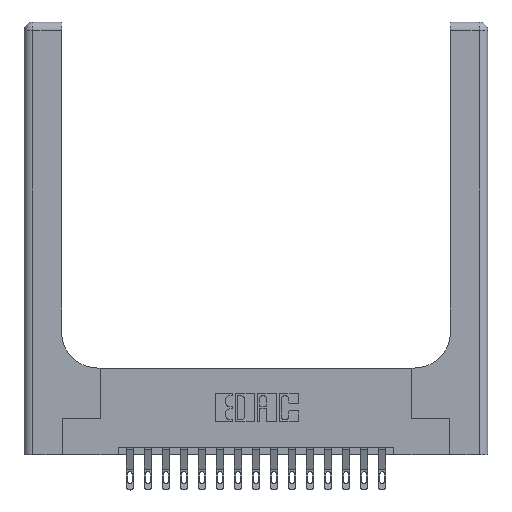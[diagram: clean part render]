
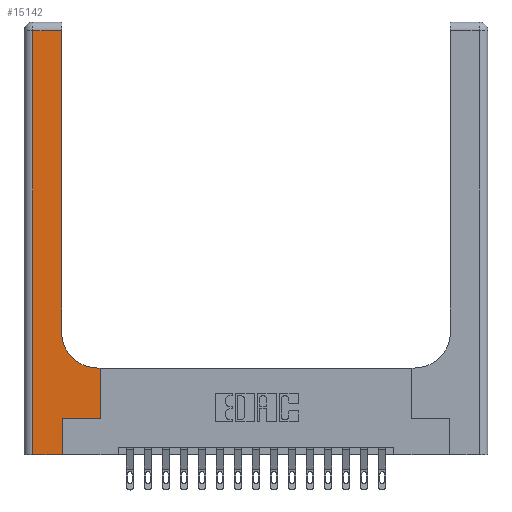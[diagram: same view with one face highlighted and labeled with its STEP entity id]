
A CAD part, top view. The second image highlights one B-rep face of the part: STEP entity #15142.
In plain terms, the highlighted planar face has unit normal (0, 0, 1).
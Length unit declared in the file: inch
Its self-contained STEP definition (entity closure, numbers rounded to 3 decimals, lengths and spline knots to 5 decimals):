
#294 = VERTEX_POINT ( 'NONE', #16903 ) ;
#1083 = CARTESIAN_POINT ( 'NONE',  ( 0.26, 2.94, 0.37 ) ) ;
#1239 = DIRECTION ( 'NONE',  ( 0., 0., -1. ) ) ;
#1346 = VECTOR ( 'NONE', #1882, 39.37008 ) ;
#1364 = CARTESIAN_POINT ( 'NONE',  ( 0.06, 0., 0.37 ) ) ;
#1372 = ORIENTED_EDGE ( 'NONE', *, *, #3000, .T. ) ;
#1452 = LINE ( 'NONE', #7087, #14960 ) ;
#1803 = DIRECTION ( 'NONE',  ( -1., 0., 0. ) ) ;
#1833 = EDGE_CURVE ( 'NONE', #3673, #9360, #3607, .T. ) ;
#1882 = DIRECTION ( 'NONE',  ( 1., 0., 0. ) ) ;
#1935 = CARTESIAN_POINT ( 'NONE',  ( 0., 3., 0.37 ) ) ;
#1961 = ORIENTED_EDGE ( 'NONE', *, *, #12701, .T. ) ;
#1982 = EDGE_CURVE ( 'NONE', #9360, #13505, #3827, .T. ) ;
#2556 = CARTESIAN_POINT ( 'NONE',  ( 0.265, 0., 0.37 ) ) ;
#2566 = VERTEX_POINT ( 'NONE', #5117 ) ;
#2608 = ORIENTED_EDGE ( 'NONE', *, *, #1982, .T. ) ;
#3000 = EDGE_CURVE ( 'NONE', #13505, #12560, #3036, .T. ) ;
#3036 = LINE ( 'NONE', #10335, #17679 ) ;
#3607 = LINE ( 'NONE', #14999, #13443 ) ;
#3612 = CARTESIAN_POINT ( 'NONE',  ( 0.06, 2.94, 0.37 ) ) ;
#3673 = VERTEX_POINT ( 'NONE', #1083 ) ;
#3827 = LINE ( 'NONE', #10155, #18252 ) ;
#4158 = DIRECTION ( 'NONE',  ( 1., 0., 0. ) ) ;
#4601 = ORIENTED_EDGE ( 'NONE', *, *, #1833, .T. ) ;
#4623 = VERTEX_POINT ( 'NONE', #6923 ) ;
#4665 = DIRECTION ( 'NONE',  ( 0., 0., -1. ) ) ;
#5117 = CARTESIAN_POINT ( 'NONE',  ( 0.51, 0.6, 0.37 ) ) ;
#5470 = DIRECTION ( 'NONE',  ( 0., 1., 0. ) ) ;
#5744 = CARTESIAN_POINT ( 'NONE',  ( 0.265, 0.25, 0.37 ) ) ;
#5911 = DIRECTION ( 'NONE',  ( 0., -1., 0. ) ) ;
#5991 = LINE ( 'NONE', #17404, #10146 ) ;
#6519 = CARTESIAN_POINT ( 'NONE',  ( 0.528, 0.25, 0.37 ) ) ;
#6750 = CIRCLE ( 'NONE', #17848, 0.25 ) ;
#6923 = CARTESIAN_POINT ( 'NONE',  ( 0.26, 0.85, 0.37 ) ) ;
#7087 = CARTESIAN_POINT ( 'NONE',  ( 0.26, 0.6, 0.37 ) ) ;
#7234 = FACE_OUTER_BOUND ( 'NONE', #9869, .T. ) ;
#7320 = DIRECTION ( 'NONE',  ( 1., 0., 0. ) ) ;
#7541 = VERTEX_POINT ( 'NONE', #16101 ) ;
#7690 = DIRECTION ( 'NONE',  ( -1., 0., 0. ) ) ;
#8969 = CARTESIAN_POINT ( 'NONE',  ( 0.265, 0.25, 0.37 ) ) ;
#9203 = ORIENTED_EDGE ( 'NONE', *, *, #15945, .T. ) ;
#9360 = VERTEX_POINT ( 'NONE', #3612 ) ;
#9620 = DIRECTION ( 'NONE',  ( 0., 1., 0. ) ) ;
#9751 = EDGE_CURVE ( 'NONE', #7541, #2566, #1452, .T. ) ;
#9777 = EDGE_CURVE ( 'NONE', #4623, #3673, #5991, .T. ) ;
#9869 = EDGE_LOOP ( 'NONE', ( #10528, #4601, #2608, #1372, #10781, #1961, #16991, #11303, #9203 ) ) ;
#10146 = VECTOR ( 'NONE', #5470, 39.37008 ) ;
#10155 = CARTESIAN_POINT ( 'NONE',  ( 0.06, 3., 0.37 ) ) ;
#10189 = VECTOR ( 'NONE', #13748, 39.37008 ) ;
#10335 = CARTESIAN_POINT ( 'NONE',  ( 0., 0., 0.37 ) ) ;
#10528 = ORIENTED_EDGE ( 'NONE', *, *, #9777, .T. ) ;
#10647 = AXIS2_PLACEMENT_3D ( 'NONE', #1935, #4665, #1803 ) ;
#10781 = ORIENTED_EDGE ( 'NONE', *, *, #12857, .T. ) ;
#11303 = ORIENTED_EDGE ( 'NONE', *, *, #9751, .T. ) ;
#12560 = VERTEX_POINT ( 'NONE', #2556 ) ;
#12701 = EDGE_CURVE ( 'NONE', #15323, #294, #13686, .T. ) ;
#12857 = EDGE_CURVE ( 'NONE', #12560, #15323, #16221, .T. ) ;
#12906 = DIRECTION ( 'NONE',  ( -1., 0., 0. ) ) ;
#12952 = CARTESIAN_POINT ( 'NONE',  ( 0.51, 0.85, 0.37 ) ) ;
#13443 = VECTOR ( 'NONE', #7690, 39.37008 ) ;
#13505 = VERTEX_POINT ( 'NONE', #1364 ) ;
#13686 = LINE ( 'NONE', #8969, #1346 ) ;
#13748 = DIRECTION ( 'NONE',  ( 0., 1., 0. ) ) ;
#13942 = VECTOR ( 'NONE', #9620, 39.37008 ) ;
#14053 = CARTESIAN_POINT ( 'NONE',  ( 0.265, 0., 0.37 ) ) ;
#14095 = LINE ( 'NONE', #6519, #10189 ) ;
#14813 = EDGE_CURVE ( 'NONE', #294, #7541, #14095, .T. ) ;
#14960 = VECTOR ( 'NONE', #12906, 39.37008 ) ;
#14999 = CARTESIAN_POINT ( 'NONE',  ( 0., 2.94, 0.37 ) ) ;
#15142 = ADVANCED_FACE ( 'NONE', ( #7234 ), #16420, .F. ) ;
#15323 = VERTEX_POINT ( 'NONE', #5744 ) ;
#15945 = EDGE_CURVE ( 'NONE', #2566, #4623, #6750, .T. ) ;
#16101 = CARTESIAN_POINT ( 'NONE',  ( 0.528, 0.6, 0.37 ) ) ;
#16221 = LINE ( 'NONE', #14053, #13942 ) ;
#16420 = PLANE ( 'NONE',  #10647 ) ;
#16903 = CARTESIAN_POINT ( 'NONE',  ( 0.528, 0.25, 0.37 ) ) ;
#16991 = ORIENTED_EDGE ( 'NONE', *, *, #14813, .T. ) ;
#17404 = CARTESIAN_POINT ( 'NONE',  ( 0.26, 3., 0.37 ) ) ;
#17679 = VECTOR ( 'NONE', #7320, 39.37008 ) ;
#17848 = AXIS2_PLACEMENT_3D ( 'NONE', #12952, #1239, #4158 ) ;
#18252 = VECTOR ( 'NONE', #5911, 39.37008 ) ;
